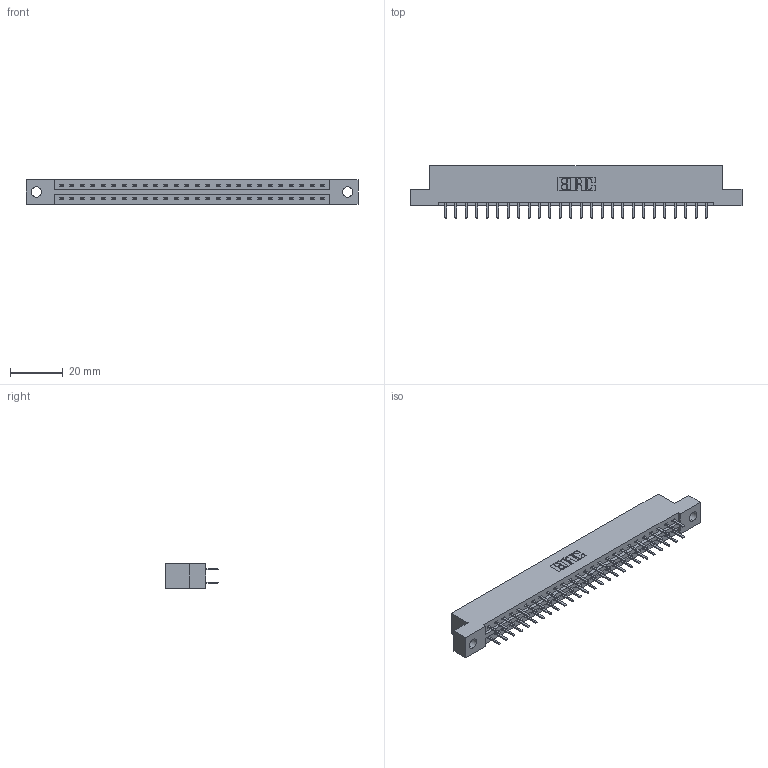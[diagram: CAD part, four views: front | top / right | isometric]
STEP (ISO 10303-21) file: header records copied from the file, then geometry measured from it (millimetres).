
FILE_DESCRIPTION (( 'STEP AP203' ), '1' );
FILE_NAME ('337-052-520-204.STEP', '2018-08-09T22:09:38', ( '' ), ( '' ), 'SwSTEP 2.0', 'SolidWorks 2016', '' );
FILE_SCHEMA (( 'CONFIG_CONTROL_DESIGN' ));
Length unit declared in the file: inch
Products named in the file (3): 337-052-520-204; 337 Part_Flush Mounting Lugs - 0.156 Dia-TH; 345-292-001_345-293-120
Assembly tree (53 placements, depth 2):
  337-052-520-204
    337 Part_Flush Mounting Lugs - 0.156 Dia-TH
    345-292-001_345-293-120  x52
Bounding box: 126.03 x 20.02 x 9.4 mm (x, y, z)
Volume: 12958.9 mm3; surface area: 14226.8 mm2
Topology: 53 solids, 53 shells, 3130 faces, 9099 edges, 5926 vertices
Faces by surface type: plane 2150, cylinder 980
Entity records: 22345 total; most frequent: CARTESIAN_POINT 3790, ORIENTED_EDGE 3714, DIRECTION 3241, EDGE_CURVE 1857, VECTOR 1725, LINE 1725, VERTEX_POINT 1234, AXIS2_PLACEMENT_3D 758
